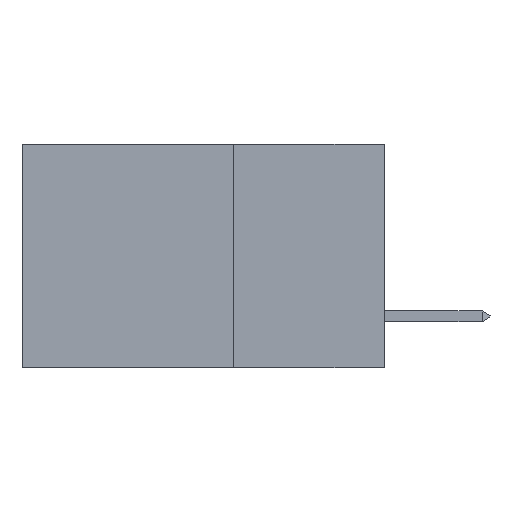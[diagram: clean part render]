
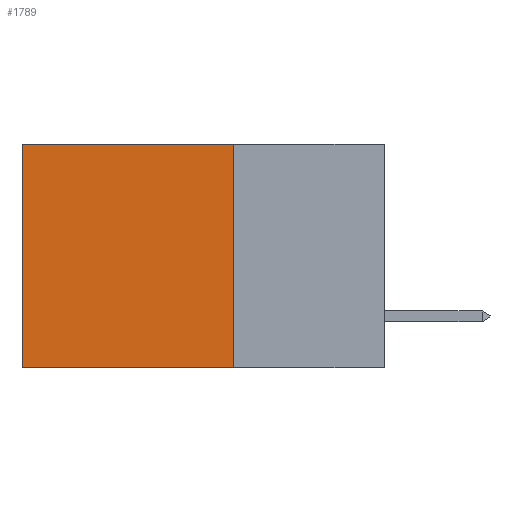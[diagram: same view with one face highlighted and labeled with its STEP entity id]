
A CAD part, left-side view. The second image highlights one B-rep face of the part: STEP entity #1789.
In plain terms, the highlighted planar face has unit normal (-1, 0, 0).
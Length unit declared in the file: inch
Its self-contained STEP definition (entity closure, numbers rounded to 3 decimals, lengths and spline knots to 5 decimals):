
#1411 = ORIENTED_EDGE ( 'NONE', *, *, #28984, .T. ) ;
#1789 = ADVANCED_FACE ( 'NONE', ( #21628 ), #18603, .F. ) ;
#2137 = CARTESIAN_POINT ( 'NONE',  ( 0.2875, 0.6, 0. ) ) ;
#4028 = LINE ( 'NONE', #34061, #22578 ) ;
#4046 = CARTESIAN_POINT ( 'NONE',  ( 0.2875, 0.25, -0.37 ) ) ;
#4221 = DIRECTION ( 'NONE',  ( 0., 1., 0. ) ) ;
#4357 = VERTEX_POINT ( 'NONE', #25434 ) ;
#5926 = ORIENTED_EDGE ( 'NONE', *, *, #14362, .F. ) ;
#5961 = EDGE_CURVE ( 'NONE', #4357, #6147, #9380, .T. ) ;
#6147 = VERTEX_POINT ( 'NONE', #32514 ) ;
#7159 = CARTESIAN_POINT ( 'NONE',  ( 0.2875, 0.6, 0. ) ) ;
#8368 = LINE ( 'NONE', #16736, #34335 ) ;
#9380 = LINE ( 'NONE', #4046, #12981 ) ;
#12144 = AXIS2_PLACEMENT_3D ( 'NONE', #35021, #29492, #21453 ) ;
#12750 = EDGE_LOOP ( 'NONE', ( #1411, #16451, #5926, #25134 ) ) ;
#12981 = VECTOR ( 'NONE', #4221, 39.37008 ) ;
#14065 = DIRECTION ( 'NONE',  ( 0., 1., 0. ) ) ;
#14362 = EDGE_CURVE ( 'NONE', #27956, #4357, #4028, .T. ) ;
#14476 = VERTEX_POINT ( 'NONE', #2137 ) ;
#16451 = ORIENTED_EDGE ( 'NONE', *, *, #5961, .F. ) ;
#16736 = CARTESIAN_POINT ( 'NONE',  ( 0.2875, 0.25, 0. ) ) ;
#17475 = VECTOR ( 'NONE', #18038, 39.37008 ) ;
#18038 = DIRECTION ( 'NONE',  ( 0., 0., -1. ) ) ;
#18603 = PLANE ( 'NONE',  #12144 ) ;
#20121 = DIRECTION ( 'NONE',  ( 0., 0., -1. ) ) ;
#21453 = DIRECTION ( 'NONE',  ( 0., 0., -1. ) ) ;
#21628 = FACE_OUTER_BOUND ( 'NONE', #12750, .T. ) ;
#22578 = VECTOR ( 'NONE', #20121, 39.37008 ) ;
#24477 = EDGE_CURVE ( 'NONE', #27956, #14476, #8368, .T. ) ;
#25134 = ORIENTED_EDGE ( 'NONE', *, *, #24477, .T. ) ;
#25434 = CARTESIAN_POINT ( 'NONE',  ( 0.2875, 0.25, -0.37 ) ) ;
#27946 = CARTESIAN_POINT ( 'NONE',  ( 0.2875, 0.25, 0. ) ) ;
#27956 = VERTEX_POINT ( 'NONE', #27946 ) ;
#28984 = EDGE_CURVE ( 'NONE', #14476, #6147, #31599, .T. ) ;
#29492 = DIRECTION ( 'NONE',  ( 1., 0., 0. ) ) ;
#31599 = LINE ( 'NONE', #7159, #17475 ) ;
#32514 = CARTESIAN_POINT ( 'NONE',  ( 0.2875, 0.6, -0.37 ) ) ;
#34061 = CARTESIAN_POINT ( 'NONE',  ( 0.2875, 0.25, 0. ) ) ;
#34335 = VECTOR ( 'NONE', #14065, 39.37008 ) ;
#35021 = CARTESIAN_POINT ( 'NONE',  ( 0.2875, 0.25, 0. ) ) ;
